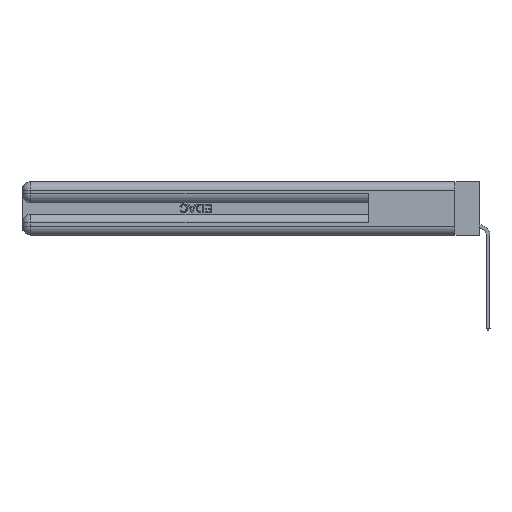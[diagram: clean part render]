
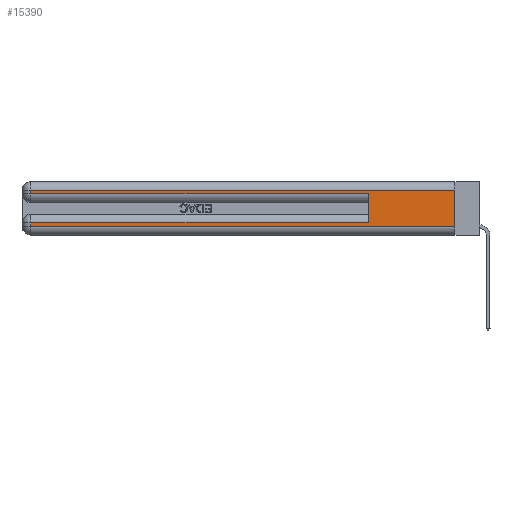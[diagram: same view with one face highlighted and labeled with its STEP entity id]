
A CAD part, left-side view. The second image highlights one B-rep face of the part: STEP entity #15390.
In plain terms, the highlighted planar face has unit normal (-1, 0, 0).
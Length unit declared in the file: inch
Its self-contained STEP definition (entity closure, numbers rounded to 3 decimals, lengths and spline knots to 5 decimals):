
#338 = CARTESIAN_POINT ( 'NONE',  ( 0., 0.6, 0.145 ) ) ;
#2221 = DIRECTION ( 'NONE',  ( 1., 0., 0. ) ) ;
#2296 = VERTEX_POINT ( 'NONE', #6157 ) ;
#2532 = DIRECTION ( 'NONE',  ( 0., 0., -1. ) ) ;
#2899 = ORIENTED_EDGE ( 'NONE', *, *, #14102, .T. ) ;
#2978 = CARTESIAN_POINT ( 'NONE',  ( 0., 0.6, 0.285 ) ) ;
#3041 = CARTESIAN_POINT ( 'NONE',  ( 0., 0., 0.31 ) ) ;
#3767 = EDGE_CURVE ( 'NONE', #10331, #2296, #27527, .T. ) ;
#3961 = VECTOR ( 'NONE', #26093, 39.37008 ) ;
#4933 = EDGE_LOOP ( 'NONE', ( #23599, #15849, #25005, #30454, #6063, #25901, #17833, #2899 ) ) ;
#5392 = DIRECTION ( 'NONE',  ( 0., 1., 0. ) ) ;
#6063 = ORIENTED_EDGE ( 'NONE', *, *, #21520, .F. ) ;
#6157 = CARTESIAN_POINT ( 'NONE',  ( 0., 2.94, 0.085 ) ) ;
#6209 = LINE ( 'NONE', #17558, #24236 ) ;
#6284 = VECTOR ( 'NONE', #9785, 39.37008 ) ;
#7019 = LINE ( 'NONE', #338, #6284 ) ;
#7044 = DIRECTION ( 'NONE',  ( 0., -1., 0. ) ) ;
#7170 = CARTESIAN_POINT ( 'NONE',  ( 0., 0., 0.37 ) ) ;
#9608 = CARTESIAN_POINT ( 'NONE',  ( 0., 0., 0.085 ) ) ;
#9785 = DIRECTION ( 'NONE',  ( 0., 0., 1. ) ) ;
#9939 = CARTESIAN_POINT ( 'NONE',  ( 0., 0.6, 0.085 ) ) ;
#10154 = VECTOR ( 'NONE', #18308, 39.37008 ) ;
#10331 = VERTEX_POINT ( 'NONE', #9939 ) ;
#10454 = FACE_OUTER_BOUND ( 'NONE', #4933, .T. ) ;
#11405 = DIRECTION ( 'NONE',  ( 0., 0., -1. ) ) ;
#11431 = LINE ( 'NONE', #30237, #17005 ) ;
#12386 = LINE ( 'NONE', #15804, #10154 ) ;
#12624 = VERTEX_POINT ( 'NONE', #24311 ) ;
#12975 = CARTESIAN_POINT ( 'NONE',  ( 0., 2.94, 0.285 ) ) ;
#13041 = VECTOR ( 'NONE', #2532, 39.37008 ) ;
#14102 = EDGE_CURVE ( 'NONE', #12624, #20122, #24152, .T. ) ;
#15390 = ADVANCED_FACE ( 'NONE', ( #10454 ), #25702, .F. ) ;
#15449 = EDGE_CURVE ( 'NONE', #15933, #20122, #19362, .T. ) ;
#15804 = CARTESIAN_POINT ( 'NONE',  ( 0., 2.94, 0.37 ) ) ;
#15849 = ORIENTED_EDGE ( 'NONE', *, *, #29845, .T. ) ;
#15933 = VERTEX_POINT ( 'NONE', #22914 ) ;
#16370 = CARTESIAN_POINT ( 'NONE',  ( 0., 0., 0.37 ) ) ;
#17005 = VECTOR ( 'NONE', #11405, 39.37008 ) ;
#17354 = DIRECTION ( 'NONE',  ( 0., -1., 0. ) ) ;
#17492 = EDGE_CURVE ( 'NONE', #28826, #19733, #12386, .T. ) ;
#17558 = CARTESIAN_POINT ( 'NONE',  ( 0., 0., 0.285 ) ) ;
#17833 = ORIENTED_EDGE ( 'NONE', *, *, #24480, .T. ) ;
#17896 = AXIS2_PLACEMENT_3D ( 'NONE', #16370, #2221, #18763 ) ;
#18308 = DIRECTION ( 'NONE',  ( 0., 0., -1. ) ) ;
#18763 = DIRECTION ( 'NONE',  ( 0., 0., -1. ) ) ;
#18841 = CARTESIAN_POINT ( 'NONE',  ( 0., 0., 0.06 ) ) ;
#19362 = LINE ( 'NONE', #7170, #13041 ) ;
#19733 = VERTEX_POINT ( 'NONE', #12975 ) ;
#20122 = VERTEX_POINT ( 'NONE', #23858 ) ;
#20264 = VERTEX_POINT ( 'NONE', #2978 ) ;
#20848 = CARTESIAN_POINT ( 'NONE',  ( 0., 2.94, 0.31 ) ) ;
#21520 = EDGE_CURVE ( 'NONE', #10331, #20264, #7019, .T. ) ;
#22914 = CARTESIAN_POINT ( 'NONE',  ( 0., 0., 0.31 ) ) ;
#22970 = VECTOR ( 'NONE', #5392, 39.37008 ) ;
#23599 = ORIENTED_EDGE ( 'NONE', *, *, #15449, .F. ) ;
#23858 = CARTESIAN_POINT ( 'NONE',  ( 0., 0., 0.06 ) ) ;
#24152 = LINE ( 'NONE', #18841, #29676 ) ;
#24236 = VECTOR ( 'NONE', #17354, 39.37008 ) ;
#24311 = CARTESIAN_POINT ( 'NONE',  ( 0., 2.94, 0.06 ) ) ;
#24480 = EDGE_CURVE ( 'NONE', #2296, #12624, #11431, .T. ) ;
#25005 = ORIENTED_EDGE ( 'NONE', *, *, #17492, .T. ) ;
#25571 = EDGE_CURVE ( 'NONE', #19733, #20264, #6209, .T. ) ;
#25702 = PLANE ( 'NONE',  #17896 ) ;
#25901 = ORIENTED_EDGE ( 'NONE', *, *, #3767, .T. ) ;
#26093 = DIRECTION ( 'NONE',  ( 0., 1., 0. ) ) ;
#27527 = LINE ( 'NONE', #9608, #3961 ) ;
#28468 = LINE ( 'NONE', #3041, #22970 ) ;
#28826 = VERTEX_POINT ( 'NONE', #20848 ) ;
#29676 = VECTOR ( 'NONE', #7044, 39.37008 ) ;
#29845 = EDGE_CURVE ( 'NONE', #15933, #28826, #28468, .T. ) ;
#30237 = CARTESIAN_POINT ( 'NONE',  ( 0., 2.94, 0.37 ) ) ;
#30454 = ORIENTED_EDGE ( 'NONE', *, *, #25571, .T. ) ;
